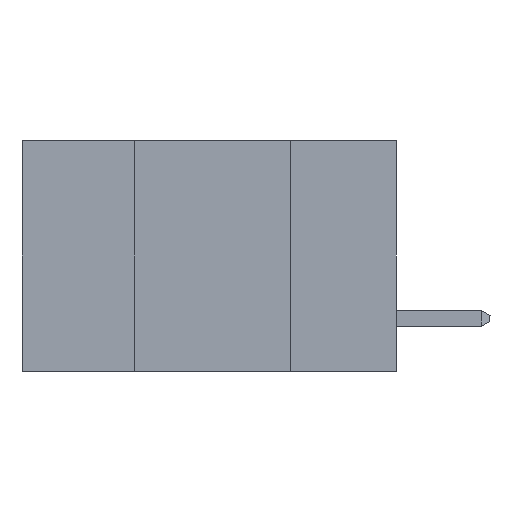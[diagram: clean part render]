
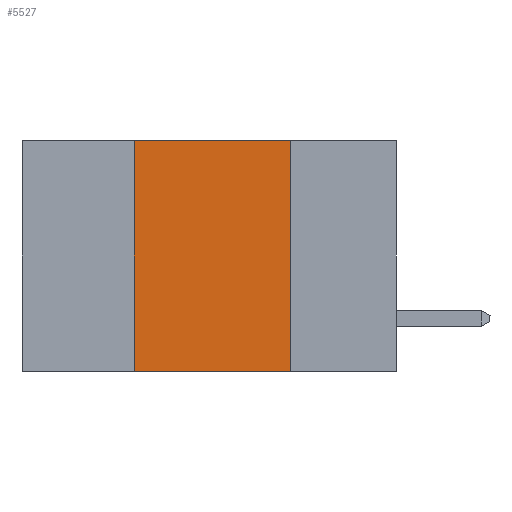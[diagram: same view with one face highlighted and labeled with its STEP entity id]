
A CAD part, left-side view. The second image highlights one B-rep face of the part: STEP entity #5527.
In plain terms, the highlighted planar face has unit normal (-1, 0, 0).
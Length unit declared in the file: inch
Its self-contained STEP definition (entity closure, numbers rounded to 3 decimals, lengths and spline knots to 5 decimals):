
#633 = LINE ( 'NONE', #10461, #4882 ) ;
#694 = EDGE_CURVE ( 'NONE', #6614, #6199, #633, .T. ) ;
#1339 = CARTESIAN_POINT ( 'NONE',  ( 0., 0.17, 0. ) ) ;
#2294 = DIRECTION ( 'NONE',  ( 0., 0., -1. ) ) ;
#3608 = VECTOR ( 'NONE', #2294, 39.37008 ) ;
#4003 = ORIENTED_EDGE ( 'NONE', *, *, #7138, .F. ) ;
#4882 = VECTOR ( 'NONE', #14500, 39.37008 ) ;
#5527 = ADVANCED_FACE ( 'NONE', ( #8369 ), #9556, .F. ) ;
#5655 = EDGE_CURVE ( 'NONE', #6614, #14353, #11556, .T. ) ;
#5873 = EDGE_CURVE ( 'NONE', #14353, #7641, #13392, .T. ) ;
#6199 = VERTEX_POINT ( 'NONE', #17584 ) ;
#6614 = VERTEX_POINT ( 'NONE', #11610 ) ;
#6986 = CARTESIAN_POINT ( 'NONE',  ( 0., 0.6, 0. ) ) ;
#7138 = EDGE_CURVE ( 'NONE', #7641, #6199, #13394, .T. ) ;
#7517 = VECTOR ( 'NONE', #14764, 39.37008 ) ;
#7641 = VERTEX_POINT ( 'NONE', #1339 ) ;
#7676 = CARTESIAN_POINT ( 'NONE',  ( 0., 0.42, 0. ) ) ;
#8258 = ORIENTED_EDGE ( 'NONE', *, *, #5873, .F. ) ;
#8369 = FACE_OUTER_BOUND ( 'NONE', #14055, .T. ) ;
#9556 = PLANE ( 'NONE',  #13961 ) ;
#10442 = VECTOR ( 'NONE', #14122, 39.37008 ) ;
#10461 = CARTESIAN_POINT ( 'NONE',  ( 0., 0.6, -0.37 ) ) ;
#11556 = LINE ( 'NONE', #14316, #10442 ) ;
#11610 = CARTESIAN_POINT ( 'NONE',  ( 0., 0.42, -0.37 ) ) ;
#13285 = CARTESIAN_POINT ( 'NONE',  ( 0., 0.6, 0. ) ) ;
#13392 = LINE ( 'NONE', #13285, #7517 ) ;
#13394 = LINE ( 'NONE', #14955, #3608 ) ;
#13961 = AXIS2_PLACEMENT_3D ( 'NONE', #6986, #15329, #15161 ) ;
#14055 = EDGE_LOOP ( 'NONE', ( #4003, #8258, #16804, #17941 ) ) ;
#14122 = DIRECTION ( 'NONE',  ( 0., 0., 1. ) ) ;
#14316 = CARTESIAN_POINT ( 'NONE',  ( 0., 0.42, -0.37 ) ) ;
#14353 = VERTEX_POINT ( 'NONE', #7676 ) ;
#14500 = DIRECTION ( 'NONE',  ( 0., -1., 0. ) ) ;
#14764 = DIRECTION ( 'NONE',  ( 0., -1., 0. ) ) ;
#14955 = CARTESIAN_POINT ( 'NONE',  ( 0., 0.17, -0.37 ) ) ;
#15161 = DIRECTION ( 'NONE',  ( 0., 0., -1. ) ) ;
#15329 = DIRECTION ( 'NONE',  ( 1., 0., 0. ) ) ;
#16804 = ORIENTED_EDGE ( 'NONE', *, *, #5655, .F. ) ;
#17584 = CARTESIAN_POINT ( 'NONE',  ( 0., 0.17, -0.37 ) ) ;
#17941 = ORIENTED_EDGE ( 'NONE', *, *, #694, .T. ) ;
